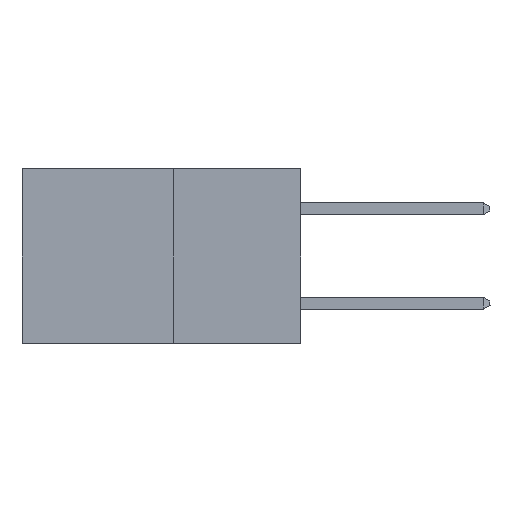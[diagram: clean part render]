
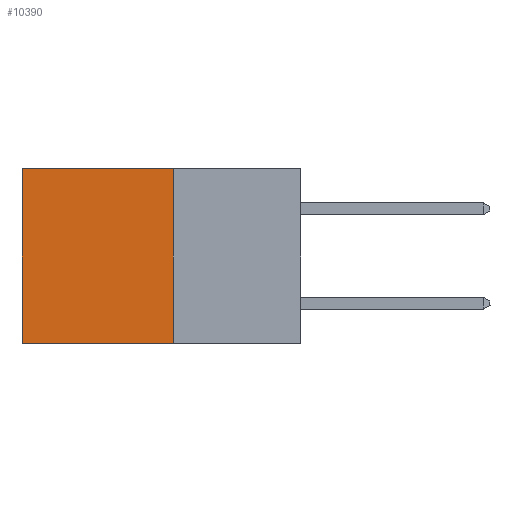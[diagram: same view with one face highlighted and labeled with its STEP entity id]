
A CAD part, left-side view. The second image highlights one B-rep face of the part: STEP entity #10390.
In plain terms, the highlighted planar face has unit normal (-1, 0, 0).
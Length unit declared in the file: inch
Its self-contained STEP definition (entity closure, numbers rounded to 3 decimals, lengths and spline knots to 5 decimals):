
#21 = EDGE_LOOP ( 'NONE', ( #26223, #23488, #17386, #602 ) ) ;
#259 = CARTESIAN_POINT ( 'NONE',  ( 0.277, 0.27, 0. ) ) ;
#602 = ORIENTED_EDGE ( 'NONE', *, *, #3790, .T. ) ;
#843 = VERTEX_POINT ( 'NONE', #7188 ) ;
#1608 = LINE ( 'NONE', #259, #11526 ) ;
#2585 = CARTESIAN_POINT ( 'NONE',  ( 0.277, 0.27, -0.37 ) ) ;
#3136 = EDGE_CURVE ( 'NONE', #14343, #16562, #16825, .T. ) ;
#3617 = VECTOR ( 'NONE', #4585, 39.37008 ) ;
#3790 = EDGE_CURVE ( 'NONE', #14343, #843, #1608, .T. ) ;
#3986 = VECTOR ( 'NONE', #7798, 39.37008 ) ;
#4585 = DIRECTION ( 'NONE',  ( 0., 0., -1. ) ) ;
#5569 = CARTESIAN_POINT ( 'NONE',  ( 0.277, 0.59, -0.37 ) ) ;
#7188 = CARTESIAN_POINT ( 'NONE',  ( 0.277, 0.59, 0. ) ) ;
#7365 = EDGE_CURVE ( 'NONE', #16562, #23509, #25997, .T. ) ;
#7798 = DIRECTION ( 'NONE',  ( 0., 0., -1. ) ) ;
#8803 = CARTESIAN_POINT ( 'NONE',  ( 0.277, 0.27, -0.37 ) ) ;
#9912 = CARTESIAN_POINT ( 'NONE',  ( 0.277, 0.59, -0.37 ) ) ;
#10390 = ADVANCED_FACE ( 'NONE', ( #13822 ), #21265, .F. ) ;
#10907 = DIRECTION ( 'NONE',  ( 1., 0., 0. ) ) ;
#11121 = DIRECTION ( 'NONE',  ( 0., 1., 0. ) ) ;
#11526 = VECTOR ( 'NONE', #11121, 39.37008 ) ;
#13674 = VECTOR ( 'NONE', #18159, 39.37008 ) ;
#13822 = FACE_OUTER_BOUND ( 'NONE', #21, .T. ) ;
#14343 = VERTEX_POINT ( 'NONE', #14749 ) ;
#14358 = AXIS2_PLACEMENT_3D ( 'NONE', #8803, #10907, #25435 ) ;
#14749 = CARTESIAN_POINT ( 'NONE',  ( 0.277, 0.27, 0. ) ) ;
#15172 = LINE ( 'NONE', #9912, #3986 ) ;
#16562 = VERTEX_POINT ( 'NONE', #2585 ) ;
#16825 = LINE ( 'NONE', #24966, #3617 ) ;
#17386 = ORIENTED_EDGE ( 'NONE', *, *, #3136, .F. ) ;
#18159 = DIRECTION ( 'NONE',  ( 0., 1., 0. ) ) ;
#21265 = PLANE ( 'NONE',  #14358 ) ;
#22313 = CARTESIAN_POINT ( 'NONE',  ( 0.277, 0.27, -0.37 ) ) ;
#23488 = ORIENTED_EDGE ( 'NONE', *, *, #7365, .F. ) ;
#23509 = VERTEX_POINT ( 'NONE', #5569 ) ;
#24966 = CARTESIAN_POINT ( 'NONE',  ( 0.277, 0.27, -0.37 ) ) ;
#25435 = DIRECTION ( 'NONE',  ( 0., 0., -1. ) ) ;
#25848 = EDGE_CURVE ( 'NONE', #843, #23509, #15172, .T. ) ;
#25997 = LINE ( 'NONE', #22313, #13674 ) ;
#26223 = ORIENTED_EDGE ( 'NONE', *, *, #25848, .T. ) ;
